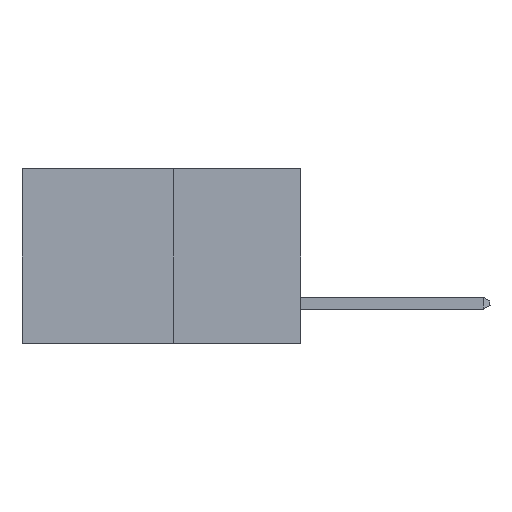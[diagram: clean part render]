
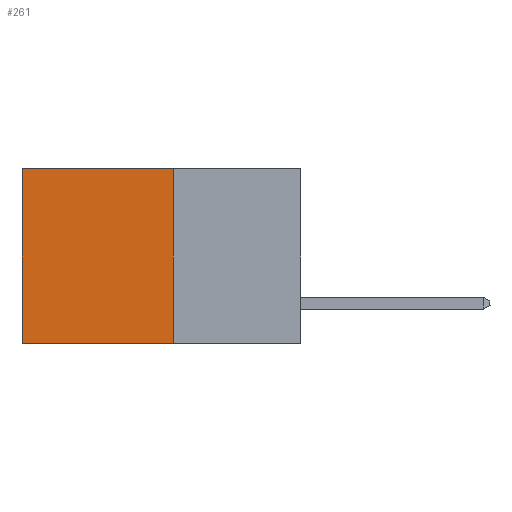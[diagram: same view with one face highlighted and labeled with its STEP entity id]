
A CAD part, left-side view. The second image highlights one B-rep face of the part: STEP entity #261.
In plain terms, the highlighted planar face has unit normal (-1, 0, 0).
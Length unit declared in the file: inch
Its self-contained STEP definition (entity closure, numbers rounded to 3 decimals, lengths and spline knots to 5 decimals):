
#261 = ADVANCED_FACE ( 'NONE', ( #1182 ), #17445, .F. ) ;
#1182 = FACE_OUTER_BOUND ( 'NONE', #3956, .T. ) ;
#1470 = CARTESIAN_POINT ( 'NONE',  ( 0.277, 0.59, -0.37 ) ) ;
#2117 = VERTEX_POINT ( 'NONE', #17760 ) ;
#2151 = EDGE_CURVE ( 'NONE', #19445, #2359, #8395, .T. ) ;
#2359 = VERTEX_POINT ( 'NONE', #14194 ) ;
#3195 = DIRECTION ( 'NONE',  ( 0., 1., 0. ) ) ;
#3510 = ORIENTED_EDGE ( 'NONE', *, *, #16396, .F. ) ;
#3833 = VECTOR ( 'NONE', #12097, 39.37008 ) ;
#3956 = EDGE_LOOP ( 'NONE', ( #9755, #6920, #3510, #5913 ) ) ;
#4638 = CARTESIAN_POINT ( 'NONE',  ( 0.277, 0.27, -0.37 ) ) ;
#5913 = ORIENTED_EDGE ( 'NONE', *, *, #13282, .T. ) ;
#6920 = ORIENTED_EDGE ( 'NONE', *, *, #2151, .F. ) ;
#7839 = VECTOR ( 'NONE', #17203, 39.37008 ) ;
#8031 = LINE ( 'NONE', #22553, #3833 ) ;
#8395 = LINE ( 'NONE', #17453, #7839 ) ;
#8678 = LINE ( 'NONE', #22606, #17519 ) ;
#8685 = VECTOR ( 'NONE', #13982, 39.37008 ) ;
#9755 = ORIENTED_EDGE ( 'NONE', *, *, #20682, .T. ) ;
#11291 = DIRECTION ( 'NONE',  ( 1., 0., 0. ) ) ;
#11912 = AXIS2_PLACEMENT_3D ( 'NONE', #4638, #11291, #17808 ) ;
#12097 = DIRECTION ( 'NONE',  ( 0., 0., -1. ) ) ;
#12381 = CARTESIAN_POINT ( 'NONE',  ( 0.277, 0.27, -0.37 ) ) ;
#13165 = VERTEX_POINT ( 'NONE', #13654 ) ;
#13282 = EDGE_CURVE ( 'NONE', #2117, #13165, #8678, .T. ) ;
#13654 = CARTESIAN_POINT ( 'NONE',  ( 0.277, 0.59, 0. ) ) ;
#13982 = DIRECTION ( 'NONE',  ( 0., 0., -1. ) ) ;
#14194 = CARTESIAN_POINT ( 'NONE',  ( 0.277, 0.59, -0.37 ) ) ;
#16396 = EDGE_CURVE ( 'NONE', #2117, #19445, #8031, .T. ) ;
#17203 = DIRECTION ( 'NONE',  ( 0., 1., 0. ) ) ;
#17445 = PLANE ( 'NONE',  #11912 ) ;
#17453 = CARTESIAN_POINT ( 'NONE',  ( 0.277, 0.27, -0.37 ) ) ;
#17519 = VECTOR ( 'NONE', #3195, 39.37008 ) ;
#17760 = CARTESIAN_POINT ( 'NONE',  ( 0.277, 0.27, 0. ) ) ;
#17808 = DIRECTION ( 'NONE',  ( 0., 0., -1. ) ) ;
#18622 = LINE ( 'NONE', #1470, #8685 ) ;
#19445 = VERTEX_POINT ( 'NONE', #12381 ) ;
#20682 = EDGE_CURVE ( 'NONE', #13165, #2359, #18622, .T. ) ;
#22553 = CARTESIAN_POINT ( 'NONE',  ( 0.277, 0.27, -0.37 ) ) ;
#22606 = CARTESIAN_POINT ( 'NONE',  ( 0.277, 0.27, 0. ) ) ;
